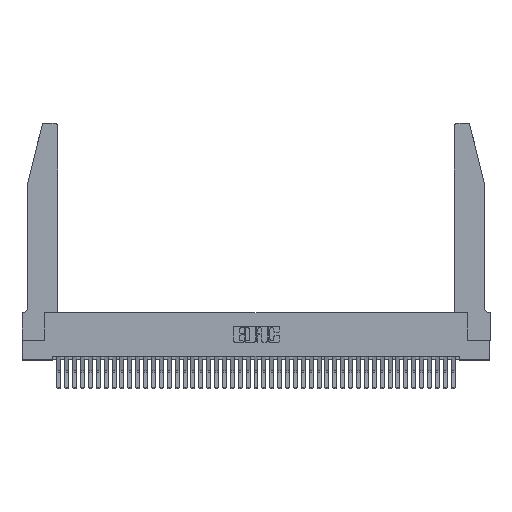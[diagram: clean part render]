
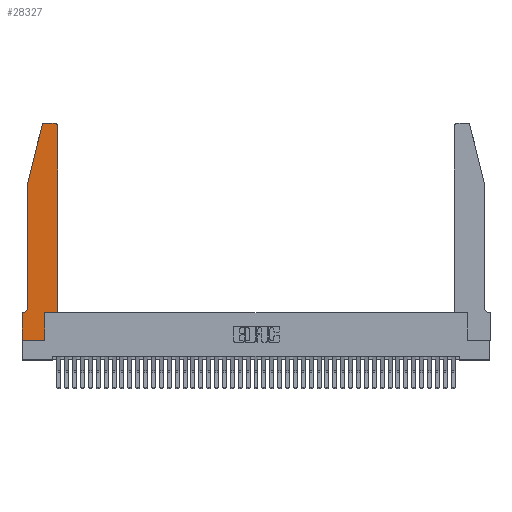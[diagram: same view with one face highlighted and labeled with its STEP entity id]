
A CAD part, top view. The second image highlights one B-rep face of the part: STEP entity #28327.
In plain terms, the highlighted planar face has unit normal (0, 0, 1).
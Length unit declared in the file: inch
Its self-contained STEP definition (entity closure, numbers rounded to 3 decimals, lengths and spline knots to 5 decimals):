
#435 = ORIENTED_EDGE ( 'NONE', *, *, #17367, .T. ) ;
#614 = CIRCLE ( 'NONE', #38103, 0.03 ) ;
#687 = CARTESIAN_POINT ( 'NONE',  ( 0.4505, 2.72, 0.37 ) ) ;
#796 = EDGE_CURVE ( 'NONE', #33396, #13808, #14044, .T. ) ;
#1168 = VECTOR ( 'NONE', #33209, 39.37008 ) ;
#1734 = CARTESIAN_POINT ( 'NONE',  ( 0.284, 2.72, 0.37 ) ) ;
#2049 = ORIENTED_EDGE ( 'NONE', *, *, #27572, .T. ) ;
#2216 = DIRECTION ( 'NONE',  ( -1., 0., 0. ) ) ;
#3184 = CARTESIAN_POINT ( 'NONE',  ( 0.284, 2.75, 0.37 ) ) ;
#3434 = CARTESIAN_POINT ( 'NONE',  ( 0.0055, 0.42, 0.37 ) ) ;
#4786 = ORIENTED_EDGE ( 'NONE', *, *, #16870, .T. ) ;
#4895 = VECTOR ( 'NONE', #34502, 39.37008 ) ;
#5213 = DIRECTION ( 'NONE',  ( 1., 0., 0. ) ) ;
#5316 = ORIENTED_EDGE ( 'NONE', *, *, #33096, .T. ) ;
#5900 = DIRECTION ( 'NONE',  ( 0., 1., 0. ) ) ;
#6900 = DIRECTION ( 'NONE',  ( -1., 0., 0. ) ) ;
#7210 = VECTOR ( 'NONE', #2216, 39.37008 ) ;
#7489 = ORIENTED_EDGE ( 'NONE', *, *, #796, .T. ) ;
#7688 = VECTOR ( 'NONE', #25206, 39.37008 ) ;
#7850 = AXIS2_PLACEMENT_3D ( 'NONE', #40196, #33691, #13594 ) ;
#8039 = CARTESIAN_POINT ( 'NONE',  ( 0.4205, 2.75, 0.37 ) ) ;
#8307 = VERTEX_POINT ( 'NONE', #3184 ) ;
#9394 = VERTEX_POINT ( 'NONE', #38791 ) ;
#10147 = PLANE ( 'NONE',  #7850 ) ;
#10625 = CARTESIAN_POINT ( 'NONE',  ( 0., 0., 0.37 ) ) ;
#10998 = VERTEX_POINT ( 'NONE', #687 ) ;
#11065 = LINE ( 'NONE', #42879, #35773 ) ;
#11196 = CIRCLE ( 'NONE', #32783, 0.03 ) ;
#11425 = LINE ( 'NONE', #23195, #1168 ) ;
#11716 = DIRECTION ( 'NONE',  ( 0., 0., 1. ) ) ;
#12317 = ORIENTED_EDGE ( 'NONE', *, *, #31427, .T. ) ;
#12905 = CARTESIAN_POINT ( 'NONE',  ( 0.4505, 0.35, 0.37 ) ) ;
#13206 = CARTESIAN_POINT ( 'NONE',  ( 0.2865, 0.35, 0.37 ) ) ;
#13387 = ORIENTED_EDGE ( 'NONE', *, *, #41738, .T. ) ;
#13594 = DIRECTION ( 'NONE',  ( 1., 0., 0. ) ) ;
#13686 = EDGE_CURVE ( 'NONE', #18572, #22613, #11425, .T. ) ;
#13808 = VERTEX_POINT ( 'NONE', #30296 ) ;
#13947 = EDGE_CURVE ( 'NONE', #10998, #25392, #614, .T. ) ;
#14044 = LINE ( 'NONE', #21089, #4895 ) ;
#14069 = DIRECTION ( 'NONE',  ( 0., -1., 0. ) ) ;
#14230 = VERTEX_POINT ( 'NONE', #13206 ) ;
#14535 = LINE ( 'NONE', #10625, #22493 ) ;
#15014 = CARTESIAN_POINT ( 'NONE',  ( 0., 0., 0.37 ) ) ;
#15902 = EDGE_LOOP ( 'NONE', ( #2049, #12317, #13387, #40065, #5316, #7489, #16571, #435, #27639, #28675, #4786, #25059 ) ) ;
#16571 = ORIENTED_EDGE ( 'NONE', *, *, #38481, .T. ) ;
#16752 = VECTOR ( 'NONE', #31557, 39.37008 ) ;
#16870 = EDGE_CURVE ( 'NONE', #9394, #10998, #43345, .T. ) ;
#17125 = EDGE_CURVE ( 'NONE', #14230, #9394, #32990, .T. ) ;
#17367 = EDGE_CURVE ( 'NONE', #29190, #39402, #41237, .T. ) ;
#18572 = VERTEX_POINT ( 'NONE', #28799 ) ;
#21089 = CARTESIAN_POINT ( 'NONE',  ( 0.0755, 0.35, 0.37 ) ) ;
#22493 = VECTOR ( 'NONE', #14069, 39.37008 ) ;
#22604 = FACE_OUTER_BOUND ( 'NONE', #15902, .T. ) ;
#22613 = VERTEX_POINT ( 'NONE', #27001 ) ;
#23195 = CARTESIAN_POINT ( 'NONE',  ( 0.0755, 2., 0.37 ) ) ;
#23633 = VECTOR ( 'NONE', #30964, 39.37008 ) ;
#23649 = LINE ( 'NONE', #41392, #16752 ) ;
#23791 = CARTESIAN_POINT ( 'NONE',  ( 0.25487, 2.72718, 0.37 ) ) ;
#24212 = AXIS2_PLACEMENT_3D ( 'NONE', #3434, #27225, #6900 ) ;
#24311 = CARTESIAN_POINT ( 'NONE',  ( 0., 0., 0.37 ) ) ;
#25059 = ORIENTED_EDGE ( 'NONE', *, *, #13947, .T. ) ;
#25206 = DIRECTION ( 'NONE',  ( 0., 1., 0. ) ) ;
#25392 = VERTEX_POINT ( 'NONE', #8039 ) ;
#25629 = DIRECTION ( 'NONE',  ( 0., 0., 1. ) ) ;
#25677 = EDGE_CURVE ( 'NONE', #39402, #14230, #11065, .T. ) ;
#25708 = CARTESIAN_POINT ( 'NONE',  ( 0.0055, 0.35, 0.37 ) ) ;
#25979 = CIRCLE ( 'NONE', #24212, 0.07 ) ;
#27001 = CARTESIAN_POINT ( 'NONE',  ( 0.0755, 0.42, 0.37 ) ) ;
#27225 = DIRECTION ( 'NONE',  ( 0., 0., -1. ) ) ;
#27572 = EDGE_CURVE ( 'NONE', #25392, #8307, #42883, .T. ) ;
#27639 = ORIENTED_EDGE ( 'NONE', *, *, #25677, .T. ) ;
#28327 = ADVANCED_FACE ( 'NONE', ( #22604 ), #10147, .T. ) ;
#28675 = ORIENTED_EDGE ( 'NONE', *, *, #17125, .T. ) ;
#28799 = CARTESIAN_POINT ( 'NONE',  ( 0.0755, 2., 0.37 ) ) ;
#29190 = VERTEX_POINT ( 'NONE', #15014 ) ;
#29684 = DIRECTION ( 'NONE',  ( 1., 0., 0. ) ) ;
#30296 = CARTESIAN_POINT ( 'NONE',  ( 0., 0.35, 0.37 ) ) ;
#30509 = VERTEX_POINT ( 'NONE', #23791 ) ;
#30964 = DIRECTION ( 'NONE',  ( 1., 0., 0. ) ) ;
#31427 = EDGE_CURVE ( 'NONE', #8307, #30509, #11196, .T. ) ;
#31557 = DIRECTION ( 'NONE',  ( -0.239, -0.971, 0. ) ) ;
#31887 = CARTESIAN_POINT ( 'NONE',  ( 0.4205, 2.72, 0.37 ) ) ;
#32783 = AXIS2_PLACEMENT_3D ( 'NONE', #1734, #25629, #5213 ) ;
#32990 = LINE ( 'NONE', #12905, #41762 ) ;
#33096 = EDGE_CURVE ( 'NONE', #22613, #33396, #25979, .T. ) ;
#33209 = DIRECTION ( 'NONE',  ( 0., -1., 0. ) ) ;
#33396 = VERTEX_POINT ( 'NONE', #25708 ) ;
#33691 = DIRECTION ( 'NONE',  ( 0., 0., 1. ) ) ;
#34502 = DIRECTION ( 'NONE',  ( -1., 0., 0. ) ) ;
#35204 = DIRECTION ( 'NONE',  ( 1., 0., 0. ) ) ;
#35773 = VECTOR ( 'NONE', #5900, 39.37008 ) ;
#35923 = CARTESIAN_POINT ( 'NONE',  ( 0.2605, 2.75, 0.37 ) ) ;
#38103 = AXIS2_PLACEMENT_3D ( 'NONE', #31887, #11716, #35204 ) ;
#38481 = EDGE_CURVE ( 'NONE', #13808, #29190, #14535, .T. ) ;
#38791 = CARTESIAN_POINT ( 'NONE',  ( 0.4505, 0.35, 0.37 ) ) ;
#39402 = VERTEX_POINT ( 'NONE', #42276 ) ;
#40065 = ORIENTED_EDGE ( 'NONE', *, *, #13686, .T. ) ;
#40196 = CARTESIAN_POINT ( 'NONE',  ( 0., 0.35, 0.37 ) ) ;
#41237 = LINE ( 'NONE', #24311, #23633 ) ;
#41392 = CARTESIAN_POINT ( 'NONE',  ( 0.0755, 2., 0.37 ) ) ;
#41681 = CARTESIAN_POINT ( 'NONE',  ( 0.4505, 0.35, 0.37 ) ) ;
#41738 = EDGE_CURVE ( 'NONE', #30509, #18572, #23649, .T. ) ;
#41762 = VECTOR ( 'NONE', #29684, 39.37008 ) ;
#42276 = CARTESIAN_POINT ( 'NONE',  ( 0.2865, 0., 0.37 ) ) ;
#42879 = CARTESIAN_POINT ( 'NONE',  ( 0.2865, 0.35, 0.37 ) ) ;
#42883 = LINE ( 'NONE', #35923, #7210 ) ;
#43345 = LINE ( 'NONE', #41681, #7688 ) ;
